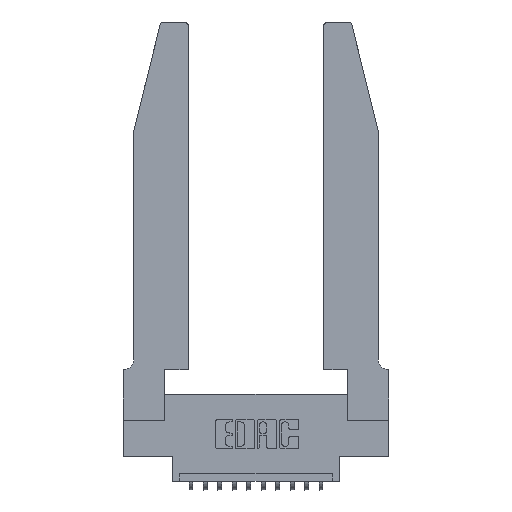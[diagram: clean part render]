
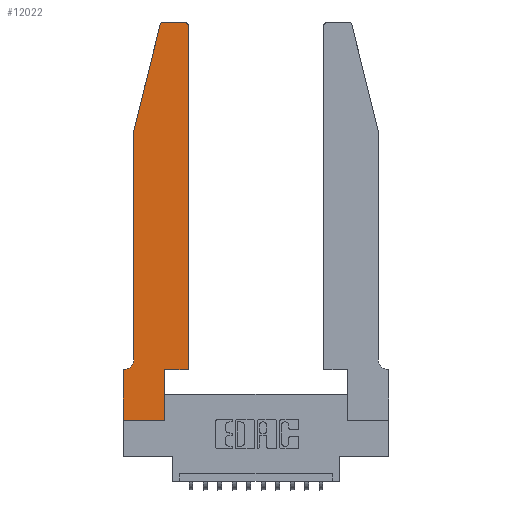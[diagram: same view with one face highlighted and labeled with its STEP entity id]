
A CAD part, top view. The second image highlights one B-rep face of the part: STEP entity #12022.
In plain terms, the highlighted planar face has unit normal (0, 0, 1).
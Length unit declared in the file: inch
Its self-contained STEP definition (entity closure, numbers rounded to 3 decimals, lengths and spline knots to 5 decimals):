
#39 = VECTOR ( 'NONE', #11726, 39.37008 ) ;
#179 = VECTOR ( 'NONE', #10420, 39.37008 ) ;
#272 = VECTOR ( 'NONE', #16727, 39.37008 ) ;
#699 = VECTOR ( 'NONE', #14823, 39.37008 ) ;
#801 = LINE ( 'NONE', #14023, #4076 ) ;
#944 = LINE ( 'NONE', #7117, #3818 ) ;
#970 = EDGE_CURVE ( 'NONE', #14281, #7531, #4237, .T. ) ;
#1025 = CARTESIAN_POINT ( 'NONE',  ( 0.2865, 0.35, 0.37 ) ) ;
#1137 = EDGE_CURVE ( 'NONE', #7531, #13439, #944, .T. ) ;
#1265 = VERTEX_POINT ( 'NONE', #4556 ) ;
#1592 = AXIS2_PLACEMENT_3D ( 'NONE', #13026, #5440, #5219 ) ;
#2020 = CARTESIAN_POINT ( 'NONE',  ( 0.4505, 2.72, 0.37 ) ) ;
#2188 = CARTESIAN_POINT ( 'NONE',  ( 0., 0., 0.37 ) ) ;
#2247 = VERTEX_POINT ( 'NONE', #10687 ) ;
#2457 = DIRECTION ( 'NONE',  ( 0., 0., 1. ) ) ;
#2947 = LINE ( 'NONE', #12008, #699 ) ;
#3059 = EDGE_CURVE ( 'NONE', #11240, #10809, #9219, .T. ) ;
#3135 = CARTESIAN_POINT ( 'NONE',  ( 0.4505, 0.35, 0.37 ) ) ;
#3509 = LINE ( 'NONE', #6189, #39 ) ;
#3535 = ORIENTED_EDGE ( 'NONE', *, *, #8019, .T. ) ;
#3766 = CIRCLE ( 'NONE', #4275, 0.03 ) ;
#3777 = DIRECTION ( 'NONE',  ( 1., 0., 0. ) ) ;
#3818 = VECTOR ( 'NONE', #8248, 39.37008 ) ;
#4076 = VECTOR ( 'NONE', #12649, 39.37008 ) ;
#4237 = LINE ( 'NONE', #13802, #16194 ) ;
#4275 = AXIS2_PLACEMENT_3D ( 'NONE', #5889, #12352, #13592 ) ;
#4458 = CARTESIAN_POINT ( 'NONE',  ( 0., 0., 0.37 ) ) ;
#4556 = CARTESIAN_POINT ( 'NONE',  ( 0.284, 2.75, 0.37 ) ) ;
#4859 = ORIENTED_EDGE ( 'NONE', *, *, #12104, .T. ) ;
#5014 = ORIENTED_EDGE ( 'NONE', *, *, #13533, .T. ) ;
#5219 = DIRECTION ( 'NONE',  ( -1., 0., 0. ) ) ;
#5388 = CARTESIAN_POINT ( 'NONE',  ( 0.0055, 0.35, 0.37 ) ) ;
#5394 = ORIENTED_EDGE ( 'NONE', *, *, #11947, .T. ) ;
#5440 = DIRECTION ( 'NONE',  ( 0., 0., -1. ) ) ;
#5461 = EDGE_LOOP ( 'NONE', ( #5394, #7719, #13741, #11386, #8595, #3535, #15468, #7954, #5014, #16814, #12435, #4859 ) ) ;
#5565 = VECTOR ( 'NONE', #8717, 39.37008 ) ;
#5889 = CARTESIAN_POINT ( 'NONE',  ( 0.284, 2.72, 0.37 ) ) ;
#6189 = CARTESIAN_POINT ( 'NONE',  ( 0.0755, 2., 0.37 ) ) ;
#6252 = CARTESIAN_POINT ( 'NONE',  ( 0., 0.35, 0.37 ) ) ;
#6356 = PLANE ( 'NONE',  #14277 ) ;
#7117 = CARTESIAN_POINT ( 'NONE',  ( 0.4505, 0.35, 0.37 ) ) ;
#7285 = LINE ( 'NONE', #1025, #10332 ) ;
#7531 = VERTEX_POINT ( 'NONE', #3135 ) ;
#7546 = CARTESIAN_POINT ( 'NONE',  ( 0., 0., 0.37 ) ) ;
#7719 = ORIENTED_EDGE ( 'NONE', *, *, #15408, .T. ) ;
#7796 = VERTEX_POINT ( 'NONE', #16733 ) ;
#7884 = EDGE_CURVE ( 'NONE', #16592, #12214, #13143, .T. ) ;
#7954 = ORIENTED_EDGE ( 'NONE', *, *, #3059, .T. ) ;
#8019 = EDGE_CURVE ( 'NONE', #12214, #7796, #2947, .T. ) ;
#8248 = DIRECTION ( 'NONE',  ( 0., 1., 0. ) ) ;
#8595 = ORIENTED_EDGE ( 'NONE', *, *, #7884, .T. ) ;
#8717 = DIRECTION ( 'NONE',  ( 1., 0., 0. ) ) ;
#9095 = CARTESIAN_POINT ( 'NONE',  ( 0.0755, 0.42, 0.37 ) ) ;
#9219 = LINE ( 'NONE', #2188, #5565 ) ;
#9497 = EDGE_CURVE ( 'NONE', #2247, #14656, #3509, .T. ) ;
#10189 = DIRECTION ( 'NONE',  ( 0., 1., 0. ) ) ;
#10332 = VECTOR ( 'NONE', #10189, 39.37008 ) ;
#10420 = DIRECTION ( 'NONE',  ( 0., -1., 0. ) ) ;
#10661 = LINE ( 'NONE', #16669, #272 ) ;
#10687 = CARTESIAN_POINT ( 'NONE',  ( 0.25487, 2.72718, 0.37 ) ) ;
#10809 = VERTEX_POINT ( 'NONE', #13820 ) ;
#11240 = VERTEX_POINT ( 'NONE', #4458 ) ;
#11386 = ORIENTED_EDGE ( 'NONE', *, *, #15620, .T. ) ;
#11500 = VERTEX_POINT ( 'NONE', #15528 ) ;
#11608 = DIRECTION ( 'NONE',  ( 0., 0., 1. ) ) ;
#11726 = DIRECTION ( 'NONE',  ( -0.239, -0.971, 0. ) ) ;
#11947 = EDGE_CURVE ( 'NONE', #11500, #1265, #801, .T. ) ;
#11997 = LINE ( 'NONE', #7546, #179 ) ;
#12008 = CARTESIAN_POINT ( 'NONE',  ( 0.0755, 0.35, 0.37 ) ) ;
#12022 = ADVANCED_FACE ( 'NONE', ( #13639 ), #6356, .T. ) ;
#12104 = EDGE_CURVE ( 'NONE', #13439, #11500, #14261, .T. ) ;
#12214 = VERTEX_POINT ( 'NONE', #5388 ) ;
#12352 = DIRECTION ( 'NONE',  ( 0., 0., 1. ) ) ;
#12435 = ORIENTED_EDGE ( 'NONE', *, *, #1137, .T. ) ;
#12547 = AXIS2_PLACEMENT_3D ( 'NONE', #15560, #11608, #13141 ) ;
#12649 = DIRECTION ( 'NONE',  ( -1., 0., 0. ) ) ;
#12710 = EDGE_CURVE ( 'NONE', #7796, #11240, #11997, .T. ) ;
#13026 = CARTESIAN_POINT ( 'NONE',  ( 0.0055, 0.42, 0.37 ) ) ;
#13038 = DIRECTION ( 'NONE',  ( 1., 0., 0. ) ) ;
#13141 = DIRECTION ( 'NONE',  ( 1., 0., 0. ) ) ;
#13143 = CIRCLE ( 'NONE', #1592, 0.07 ) ;
#13439 = VERTEX_POINT ( 'NONE', #2020 ) ;
#13533 = EDGE_CURVE ( 'NONE', #10809, #14281, #7285, .T. ) ;
#13592 = DIRECTION ( 'NONE',  ( 1., 0., 0. ) ) ;
#13639 = FACE_OUTER_BOUND ( 'NONE', #5461, .T. ) ;
#13741 = ORIENTED_EDGE ( 'NONE', *, *, #9497, .T. ) ;
#13802 = CARTESIAN_POINT ( 'NONE',  ( 0.4505, 0.35, 0.37 ) ) ;
#13820 = CARTESIAN_POINT ( 'NONE',  ( 0.2865, 0., 0.37 ) ) ;
#13936 = CARTESIAN_POINT ( 'NONE',  ( 0.0755, 2., 0.37 ) ) ;
#14023 = CARTESIAN_POINT ( 'NONE',  ( 0.2605, 2.75, 0.37 ) ) ;
#14261 = CIRCLE ( 'NONE', #12547, 0.03 ) ;
#14277 = AXIS2_PLACEMENT_3D ( 'NONE', #6252, #2457, #3777 ) ;
#14281 = VERTEX_POINT ( 'NONE', #14495 ) ;
#14495 = CARTESIAN_POINT ( 'NONE',  ( 0.2865, 0.35, 0.37 ) ) ;
#14656 = VERTEX_POINT ( 'NONE', #13936 ) ;
#14823 = DIRECTION ( 'NONE',  ( -1., 0., 0. ) ) ;
#15408 = EDGE_CURVE ( 'NONE', #1265, #2247, #3766, .T. ) ;
#15468 = ORIENTED_EDGE ( 'NONE', *, *, #12710, .T. ) ;
#15528 = CARTESIAN_POINT ( 'NONE',  ( 0.4205, 2.75, 0.37 ) ) ;
#15560 = CARTESIAN_POINT ( 'NONE',  ( 0.4205, 2.72, 0.37 ) ) ;
#15620 = EDGE_CURVE ( 'NONE', #14656, #16592, #10661, .T. ) ;
#16194 = VECTOR ( 'NONE', #13038, 39.37008 ) ;
#16592 = VERTEX_POINT ( 'NONE', #9095 ) ;
#16669 = CARTESIAN_POINT ( 'NONE',  ( 0.0755, 2., 0.37 ) ) ;
#16727 = DIRECTION ( 'NONE',  ( 0., -1., 0. ) ) ;
#16733 = CARTESIAN_POINT ( 'NONE',  ( 0., 0.35, 0.37 ) ) ;
#16814 = ORIENTED_EDGE ( 'NONE', *, *, #970, .T. ) ;
